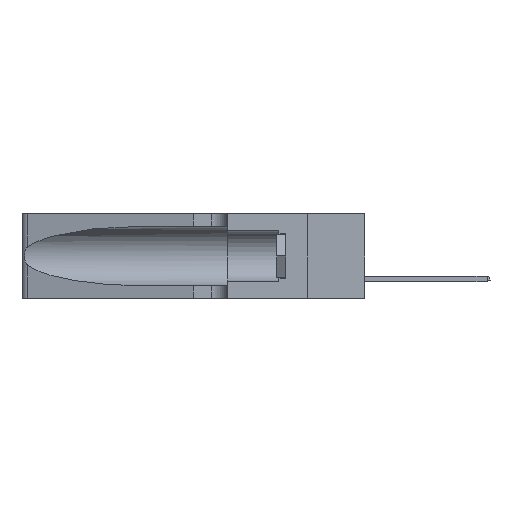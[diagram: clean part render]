
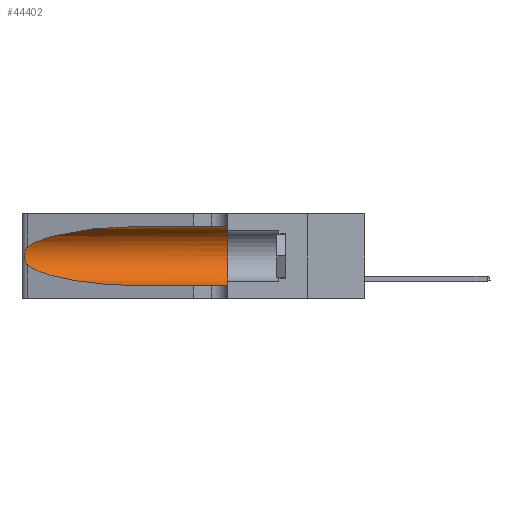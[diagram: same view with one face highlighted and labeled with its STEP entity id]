
A CAD part, left-side view. The second image highlights one B-rep face of the part: STEP entity #44402.
In plain terms, the highlighted cylindrical face has radius 3.308 mm (diameter 6.617 mm), a partial arc.
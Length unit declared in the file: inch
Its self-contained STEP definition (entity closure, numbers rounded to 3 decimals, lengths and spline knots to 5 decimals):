
#979 = CARTESIAN_POINT ( 'NONE',  ( 0.2373, 1.15595, 0.28018 ) ) ;
#1842 = CARTESIAN_POINT ( 'NONE',  ( 0.1305, 0.35, 0.185 ) ) ;
#4992 =( BOUNDED_CURVE ( )  B_SPLINE_CURVE ( 3, ( #7821, #11639, #979, #17312 ),
 .UNSPECIFIED., .F., .F. ) 
 B_SPLINE_CURVE_WITH_KNOTS ( ( 4, 4 ),
 ( 1.5708, 2.84003 ),
 .UNSPECIFIED. ) 
 CURVE ( )  GEOMETRIC_REPRESENTATION_ITEM ( )  RATIONAL_B_SPLINE_CURVE ( ( 1., 0.87, 0.87, 1. ) ) 
 REPRESENTATION_ITEM ( '' )  );
#6452 = CARTESIAN_POINT ( 'NONE',  ( 0.25789, 1.23486, 0.15765 ) ) ;
#6604 =( BOUNDED_CURVE ( )  B_SPLINE_CURVE ( 3, ( #25704, #17595, #21655, #17238 ),
 .UNSPECIFIED., .F., .F. ) 
 B_SPLINE_CURVE_WITH_KNOTS ( ( 4, 4 ),
 ( 3.44316, 4.71239 ),
 .UNSPECIFIED. ) 
 CURVE ( )  GEOMETRIC_REPRESENTATION_ITEM ( )  RATIONAL_B_SPLINE_CURVE ( ( 1., 0.87, 0.87, 1. ) ) 
 REPRESENTATION_ITEM ( '' )  );
#6729 = CARTESIAN_POINT ( 'NONE',  ( 0.1305, 1.61858, 0.05475 ) ) ;
#7821 = CARTESIAN_POINT ( 'NONE',  ( 0.1305, 0.72297, 0.31525 ) ) ;
#7901 = CARTESIAN_POINT ( 'NONE',  ( 0.25487, 1.22718, 0.14631 ) ) ;
#8590 = CARTESIAN_POINT ( 'NONE',  ( 0.26075, 1.23896, 0.19203 ) ) ;
#11348 = EDGE_CURVE ( 'NONE', #34691, #36456, #31310, .T. ) ;
#11639 = CARTESIAN_POINT ( 'NONE',  ( 0.18966, 0.96281, 0.31525 ) ) ;
#12592 = CARTESIAN_POINT ( 'NONE',  ( 0.26018, 1.23835, 0.19895 ) ) ;
#14043 = CARTESIAN_POINT ( 'NONE',  ( 0.1305, 1.61858, 0.185 ) ) ;
#17238 = CARTESIAN_POINT ( 'NONE',  ( 0.1305, 0.72297, 0.05475 ) ) ;
#17312 = CARTESIAN_POINT ( 'NONE',  ( 0.25487, 1.22718, 0.22369 ) ) ;
#17424 = DIRECTION ( 'NONE',  ( 0., -1., 0. ) ) ;
#17595 = CARTESIAN_POINT ( 'NONE',  ( 0.2373, 1.15595, 0.08982 ) ) ;
#17861 = CARTESIAN_POINT ( 'NONE',  ( 0.25639, 1.23186, 0.15144 ) ) ;
#18002 = CARTESIAN_POINT ( 'NONE',  ( 0.25487, 1.22718, 0.22369 ) ) ;
#19244 = AXIS2_PLACEMENT_3D ( 'NONE', #14043, #41213, #22323 ) ;
#19786 = B_SPLINE_CURVE_WITH_KNOTS ( 'NONE', 3,
 ( #31269, #39031, #48121, #29617, #29955, #12592, #8590, #47485, #28783, #36888, #6452, #17861, #33726, #31824 ),
 .UNSPECIFIED., .F., .F.,
 ( 4, 2, 2, 2, 2, 2, 4 ),
 ( 0., 0.00027, 0.00053, 0.00107, 0.0016, 0.00187, 0.00214 ),
 .UNSPECIFIED. ) ;
#21555 = EDGE_CURVE ( 'NONE', #22634, #49123, #27789, .T. ) ;
#21655 = CARTESIAN_POINT ( 'NONE',  ( 0.18966, 0.96281, 0.05475 ) ) ;
#21845 = AXIS2_PLACEMENT_3D ( 'NONE', #1842, #25257, #28929 ) ;
#22323 = DIRECTION ( 'NONE',  ( 0., 0., -1. ) ) ;
#22634 = VERTEX_POINT ( 'NONE', #25021 ) ;
#22674 = CYLINDRICAL_SURFACE ( 'NONE', #19244, 0.13025 ) ;
#24567 = ORIENTED_EDGE ( 'NONE', *, *, #33069, .T. ) ;
#24794 = EDGE_CURVE ( 'NONE', #34691, #26711, #4992, .T. ) ;
#25021 = CARTESIAN_POINT ( 'NONE',  ( 0.1305, 0.72297, 0.05475 ) ) ;
#25257 = DIRECTION ( 'NONE',  ( 0., 1., 0. ) ) ;
#25704 = CARTESIAN_POINT ( 'NONE',  ( 0.25487, 1.22718, 0.14631 ) ) ;
#26428 = VERTEX_POINT ( 'NONE', #7901 ) ;
#26613 = VECTOR ( 'NONE', #48307, 39.37008 ) ;
#26711 = VERTEX_POINT ( 'NONE', #18002 ) ;
#27789 = LINE ( 'NONE', #6729, #37495 ) ;
#28783 = CARTESIAN_POINT ( 'NONE',  ( 0.26017, 1.23833, 0.17102 ) ) ;
#28929 = DIRECTION ( 'NONE',  ( 0., 0., 1. ) ) ;
#29266 = CARTESIAN_POINT ( 'NONE',  ( 0.1305, 1.61858, 0.31525 ) ) ;
#29617 = CARTESIAN_POINT ( 'NONE',  ( 0.25787, 1.23484, 0.2124 ) ) ;
#29955 = CARTESIAN_POINT ( 'NONE',  ( 0.25854, 1.2359, 0.20912 ) ) ;
#30304 = ORIENTED_EDGE ( 'NONE', *, *, #11348, .F. ) ;
#30350 = ORIENTED_EDGE ( 'NONE', *, *, #35591, .T. ) ;
#31269 = CARTESIAN_POINT ( 'NONE',  ( 0.25487, 1.22718, 0.22369 ) ) ;
#31310 = LINE ( 'NONE', #29266, #26613 ) ;
#31638 = CARTESIAN_POINT ( 'NONE',  ( 0.1305, 0.72297, 0.31525 ) ) ;
#31686 = CIRCLE ( 'NONE', #21845, 0.13025 ) ;
#31824 = CARTESIAN_POINT ( 'NONE',  ( 0.25487, 1.22718, 0.14631 ) ) ;
#33069 = EDGE_CURVE ( 'NONE', #26428, #22634, #6604, .T. ) ;
#33657 = CARTESIAN_POINT ( 'NONE',  ( 0.1305, 0.35, 0.05475 ) ) ;
#33726 = CARTESIAN_POINT ( 'NONE',  ( 0.25555, 1.22993, 0.14849 ) ) ;
#34691 = VERTEX_POINT ( 'NONE', #31638 ) ;
#35591 = EDGE_CURVE ( 'NONE', #26711, #26428, #19786, .T. ) ;
#36456 = VERTEX_POINT ( 'NONE', #48155 ) ;
#36473 = FACE_OUTER_BOUND ( 'NONE', #37021, .T. ) ;
#36888 = CARTESIAN_POINT ( 'NONE',  ( 0.25856, 1.23593, 0.16098 ) ) ;
#37021 = EDGE_LOOP ( 'NONE', ( #37586, #30350, #24567, #45769, #42783, #30304 ) ) ;
#37495 = VECTOR ( 'NONE', #17424, 39.37008 ) ;
#37586 = ORIENTED_EDGE ( 'NONE', *, *, #24794, .T. ) ;
#39031 = CARTESIAN_POINT ( 'NONE',  ( 0.25555, 1.22994, 0.2215 ) ) ;
#41213 = DIRECTION ( 'NONE',  ( 0., -1., 0. ) ) ;
#42783 = ORIENTED_EDGE ( 'NONE', *, *, #43948, .F. ) ;
#43948 = EDGE_CURVE ( 'NONE', #36456, #49123, #31686, .T. ) ;
#44402 = ADVANCED_FACE ( 'NONE', ( #36473 ), #22674, .F. ) ;
#45769 = ORIENTED_EDGE ( 'NONE', *, *, #21555, .T. ) ;
#47485 = CARTESIAN_POINT ( 'NONE',  ( 0.26075, 1.23896, 0.178 ) ) ;
#48121 = CARTESIAN_POINT ( 'NONE',  ( 0.25639, 1.23184, 0.21858 ) ) ;
#48155 = CARTESIAN_POINT ( 'NONE',  ( 0.1305, 0.35, 0.31525 ) ) ;
#48307 = DIRECTION ( 'NONE',  ( 0., -1., 0. ) ) ;
#49123 = VERTEX_POINT ( 'NONE', #33657 ) ;
